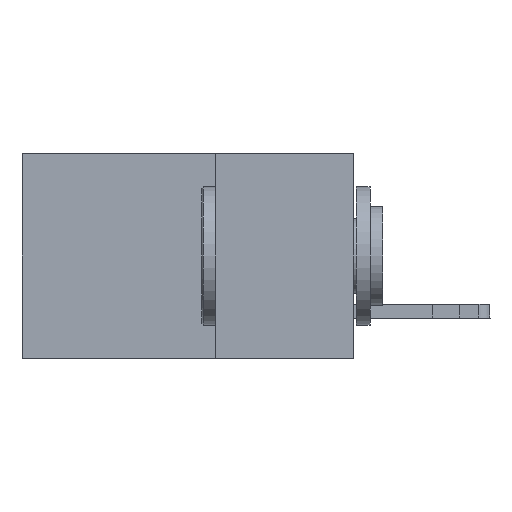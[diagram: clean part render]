
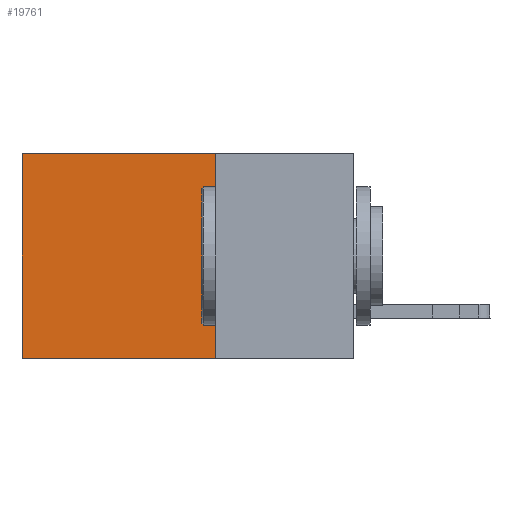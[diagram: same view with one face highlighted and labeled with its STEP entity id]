
A CAD part, left-side view. The second image highlights one B-rep face of the part: STEP entity #19761.
In plain terms, the highlighted planar face has unit normal (-1, 0, 0).
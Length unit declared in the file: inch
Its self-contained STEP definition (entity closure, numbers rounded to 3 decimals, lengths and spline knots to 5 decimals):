
#1202 = ORIENTED_EDGE ( 'NONE', *, *, #15121, .F. ) ;
#1496 = CARTESIAN_POINT ( 'NONE',  ( 0.2875, 0.6, 0. ) ) ;
#1497 = CARTESIAN_POINT ( 'NONE',  ( 0.2875, 0.6, -0.37 ) ) ;
#1703 = CARTESIAN_POINT ( 'NONE',  ( 0.2875, 0.25, 0. ) ) ;
#1706 = DIRECTION ( 'NONE',  ( 0., 1., 0. ) ) ;
#2068 = DIRECTION ( 'NONE',  ( 0., 1., 0. ) ) ;
#3012 = VERTEX_POINT ( 'NONE', #26574 ) ;
#3829 = CARTESIAN_POINT ( 'NONE',  ( 0.2875, 0.6, 0. ) ) ;
#4633 = VECTOR ( 'NONE', #1706, 39.37008 ) ;
#6193 = PLANE ( 'NONE',  #11407 ) ;
#6640 = CARTESIAN_POINT ( 'NONE',  ( 0.2875, 0.25, 0. ) ) ;
#6864 = EDGE_CURVE ( 'NONE', #9212, #21504, #22039, .T. ) ;
#8343 = EDGE_CURVE ( 'NONE', #3012, #26488, #9345, .T. ) ;
#9212 = VERTEX_POINT ( 'NONE', #3829 ) ;
#9345 = LINE ( 'NONE', #6640, #27984 ) ;
#10270 = ORIENTED_EDGE ( 'NONE', *, *, #12300, .T. ) ;
#10487 = DIRECTION ( 'NONE',  ( 0., 0., -1. ) ) ;
#11199 = LINE ( 'NONE', #21987, #28456 ) ;
#11407 = AXIS2_PLACEMENT_3D ( 'NONE', #1703, #23951, #10487 ) ;
#12300 = EDGE_CURVE ( 'NONE', #3012, #9212, #11199, .T. ) ;
#12416 = FACE_OUTER_BOUND ( 'NONE', #26823, .T. ) ;
#15121 = EDGE_CURVE ( 'NONE', #26488, #21504, #24312, .T. ) ;
#18370 = ORIENTED_EDGE ( 'NONE', *, *, #8343, .F. ) ;
#19219 = VECTOR ( 'NONE', #23928, 39.37008 ) ;
#19761 = ADVANCED_FACE ( 'NONE', ( #12416 ), #6193, .F. ) ;
#20005 = CARTESIAN_POINT ( 'NONE',  ( 0.2875, 0.25, -0.37 ) ) ;
#21504 = VERTEX_POINT ( 'NONE', #1497 ) ;
#21987 = CARTESIAN_POINT ( 'NONE',  ( 0.2875, 0.25, 0. ) ) ;
#22039 = LINE ( 'NONE', #1496, #19219 ) ;
#22883 = ORIENTED_EDGE ( 'NONE', *, *, #6864, .T. ) ;
#23928 = DIRECTION ( 'NONE',  ( 0., 0., -1. ) ) ;
#23951 = DIRECTION ( 'NONE',  ( 1., 0., 0. ) ) ;
#24110 = DIRECTION ( 'NONE',  ( 0., 0., -1. ) ) ;
#24312 = LINE ( 'NONE', #27559, #4633 ) ;
#26488 = VERTEX_POINT ( 'NONE', #20005 ) ;
#26574 = CARTESIAN_POINT ( 'NONE',  ( 0.2875, 0.25, 0. ) ) ;
#26823 = EDGE_LOOP ( 'NONE', ( #22883, #1202, #18370, #10270 ) ) ;
#27559 = CARTESIAN_POINT ( 'NONE',  ( 0.2875, 0.25, -0.37 ) ) ;
#27984 = VECTOR ( 'NONE', #24110, 39.37008 ) ;
#28456 = VECTOR ( 'NONE', #2068, 39.37008 ) ;
